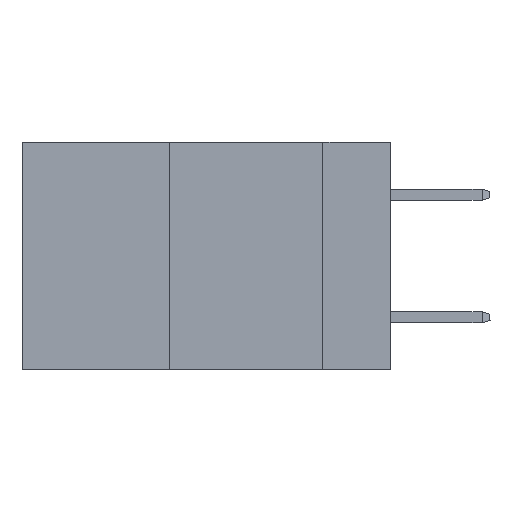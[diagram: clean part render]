
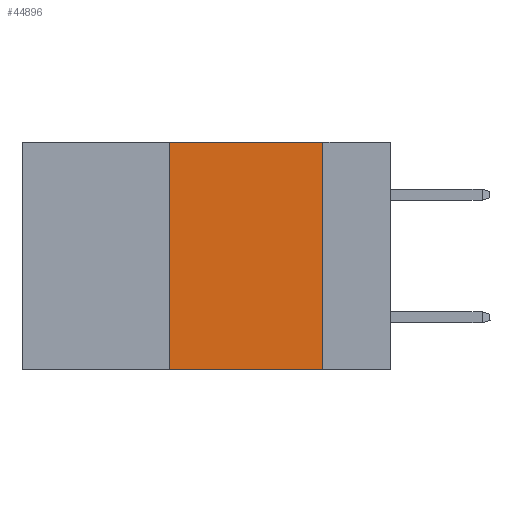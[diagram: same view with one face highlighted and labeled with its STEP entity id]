
A CAD part, left-side view. The second image highlights one B-rep face of the part: STEP entity #44896.
In plain terms, the highlighted planar face has unit normal (-1, 0, 0).
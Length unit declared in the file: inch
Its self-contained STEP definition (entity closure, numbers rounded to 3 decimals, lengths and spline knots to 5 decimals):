
#1779 = DIRECTION ( 'NONE',  ( 0., -1., 0. ) ) ;
#1830 = EDGE_CURVE ( 'NONE', #35182, #8436, #40900, .T. ) ;
#2905 = DIRECTION ( 'NONE',  ( 0., -1., 0. ) ) ;
#3115 = FACE_OUTER_BOUND ( 'NONE', #22841, .T. ) ;
#4232 = LINE ( 'NONE', #28196, #12733 ) ;
#4426 = CARTESIAN_POINT ( 'NONE',  ( 0., 0.11, 0. ) ) ;
#6006 = DIRECTION ( 'NONE',  ( 0., 0., -1. ) ) ;
#6040 = DIRECTION ( 'NONE',  ( 0., 0., 1. ) ) ;
#8436 = VERTEX_POINT ( 'NONE', #32406 ) ;
#8585 = VERTEX_POINT ( 'NONE', #18845 ) ;
#11741 = ORIENTED_EDGE ( 'NONE', *, *, #12419, .T. ) ;
#12419 = EDGE_CURVE ( 'NONE', #34721, #8436, #37777, .T. ) ;
#12733 = VECTOR ( 'NONE', #2905, 39.37008 ) ;
#12910 = ORIENTED_EDGE ( 'NONE', *, *, #30666, .F. ) ;
#15956 = ORIENTED_EDGE ( 'NONE', *, *, #29374, .F. ) ;
#18845 = CARTESIAN_POINT ( 'NONE',  ( 0., 0.36, 0. ) ) ;
#22841 = EDGE_LOOP ( 'NONE', ( #40846, #12910, #15956, #11741 ) ) ;
#24008 = CARTESIAN_POINT ( 'NONE',  ( 0., 0.6, 0. ) ) ;
#27411 = CARTESIAN_POINT ( 'NONE',  ( 0., 0.36, -0.37 ) ) ;
#27639 = DIRECTION ( 'NONE',  ( 1., 0., 0. ) ) ;
#28196 = CARTESIAN_POINT ( 'NONE',  ( 0., 0.6, 0. ) ) ;
#28967 = DIRECTION ( 'NONE',  ( 0., 0., -1. ) ) ;
#29374 = EDGE_CURVE ( 'NONE', #34721, #8585, #30690, .T. ) ;
#30666 = EDGE_CURVE ( 'NONE', #8585, #35182, #4232, .T. ) ;
#30690 = LINE ( 'NONE', #41987, #40259 ) ;
#31319 = VECTOR ( 'NONE', #28967, 39.37008 ) ;
#32406 = CARTESIAN_POINT ( 'NONE',  ( 0., 0.11, -0.37 ) ) ;
#34721 = VERTEX_POINT ( 'NONE', #27411 ) ;
#35182 = VERTEX_POINT ( 'NONE', #4426 ) ;
#36032 = CARTESIAN_POINT ( 'NONE',  ( 0., 0.11, 0. ) ) ;
#36646 = VECTOR ( 'NONE', #1779, 39.37008 ) ;
#37777 = LINE ( 'NONE', #43260, #36646 ) ;
#40259 = VECTOR ( 'NONE', #6040, 39.37008 ) ;
#40846 = ORIENTED_EDGE ( 'NONE', *, *, #1830, .F. ) ;
#40900 = LINE ( 'NONE', #36032, #31319 ) ;
#41987 = CARTESIAN_POINT ( 'NONE',  ( 0., 0.36, 0. ) ) ;
#43260 = CARTESIAN_POINT ( 'NONE',  ( 0., 0.6, -0.37 ) ) ;
#44737 = AXIS2_PLACEMENT_3D ( 'NONE', #24008, #27639, #6006 ) ;
#44896 = ADVANCED_FACE ( 'NONE', ( #3115 ), #45544, .F. ) ;
#45544 = PLANE ( 'NONE',  #44737 ) ;
